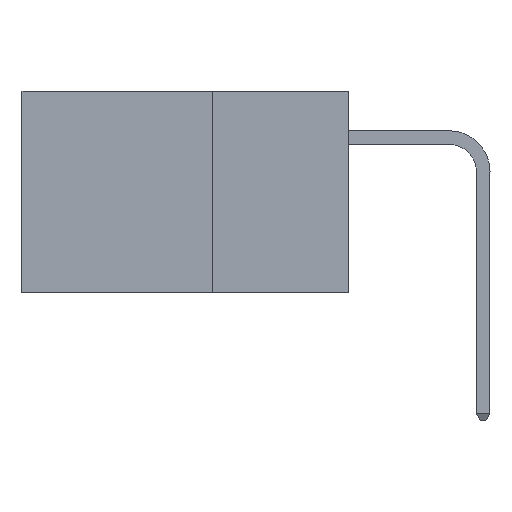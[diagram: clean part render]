
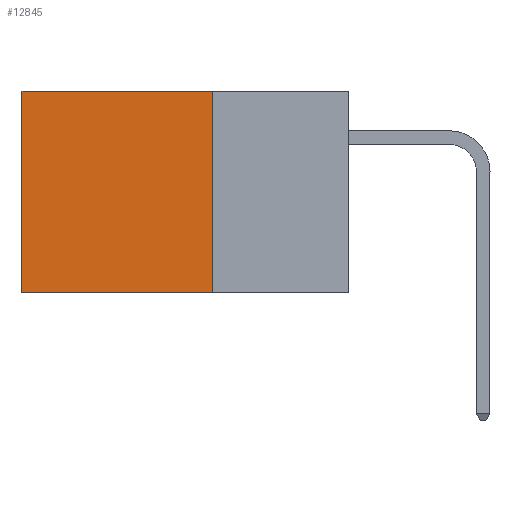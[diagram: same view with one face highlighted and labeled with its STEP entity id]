
A CAD part, left-side view. The second image highlights one B-rep face of the part: STEP entity #12845.
In plain terms, the highlighted planar face has unit normal (-1, 0, 0).
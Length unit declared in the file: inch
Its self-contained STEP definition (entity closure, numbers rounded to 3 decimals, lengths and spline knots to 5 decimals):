
#63 = LINE ( 'NONE', #13773, #2975 ) ;
#496 = DIRECTION ( 'NONE',  ( 0., 0., -1. ) ) ;
#1422 = VERTEX_POINT ( 'NONE', #14630 ) ;
#1431 = CARTESIAN_POINT ( 'NONE',  ( 0.2875, 0.25, 0. ) ) ;
#1717 = VERTEX_POINT ( 'NONE', #9365 ) ;
#2301 = PLANE ( 'NONE',  #8598 ) ;
#2401 = EDGE_CURVE ( 'NONE', #10542, #1717, #6745, .T. ) ;
#2464 = DIRECTION ( 'NONE',  ( 0., 1., 0. ) ) ;
#2975 = VECTOR ( 'NONE', #12651, 39.37008 ) ;
#3568 = DIRECTION ( 'NONE',  ( 0., 0., -1. ) ) ;
#4400 = LINE ( 'NONE', #12216, #13620 ) ;
#4548 = CARTESIAN_POINT ( 'NONE',  ( 0.2875, 0.6, 0. ) ) ;
#4964 = ORIENTED_EDGE ( 'NONE', *, *, #2401, .T. ) ;
#5554 = EDGE_CURVE ( 'NONE', #11391, #10542, #63, .T. ) ;
#5913 = CARTESIAN_POINT ( 'NONE',  ( 0.2875, 0.6, 0. ) ) ;
#6288 = ORIENTED_EDGE ( 'NONE', *, *, #10672, .F. ) ;
#6574 = VECTOR ( 'NONE', #10638, 39.37008 ) ;
#6745 = LINE ( 'NONE', #4548, #6574 ) ;
#6969 = ORIENTED_EDGE ( 'NONE', *, *, #9859, .F. ) ;
#7053 = ORIENTED_EDGE ( 'NONE', *, *, #5554, .T. ) ;
#7103 = VECTOR ( 'NONE', #496, 39.37008 ) ;
#7979 = CARTESIAN_POINT ( 'NONE',  ( 0.2875, 0.25, 0. ) ) ;
#8598 = AXIS2_PLACEMENT_3D ( 'NONE', #12011, #10877, #3568 ) ;
#9365 = CARTESIAN_POINT ( 'NONE',  ( 0.2875, 0.6, -0.37 ) ) ;
#9859 = EDGE_CURVE ( 'NONE', #11391, #1422, #13813, .T. ) ;
#10542 = VERTEX_POINT ( 'NONE', #5913 ) ;
#10638 = DIRECTION ( 'NONE',  ( 0., 0., -1. ) ) ;
#10672 = EDGE_CURVE ( 'NONE', #1422, #1717, #4400, .T. ) ;
#10877 = DIRECTION ( 'NONE',  ( 1., 0., 0. ) ) ;
#11391 = VERTEX_POINT ( 'NONE', #1431 ) ;
#12011 = CARTESIAN_POINT ( 'NONE',  ( 0.2875, 0.25, 0. ) ) ;
#12216 = CARTESIAN_POINT ( 'NONE',  ( 0.2875, 0.25, -0.37 ) ) ;
#12651 = DIRECTION ( 'NONE',  ( 0., 1., 0. ) ) ;
#12845 = ADVANCED_FACE ( 'NONE', ( #15487 ), #2301, .F. ) ;
#13620 = VECTOR ( 'NONE', #2464, 39.37008 ) ;
#13773 = CARTESIAN_POINT ( 'NONE',  ( 0.2875, 0.25, 0. ) ) ;
#13813 = LINE ( 'NONE', #7979, #7103 ) ;
#14007 = EDGE_LOOP ( 'NONE', ( #4964, #6288, #6969, #7053 ) ) ;
#14630 = CARTESIAN_POINT ( 'NONE',  ( 0.2875, 0.25, -0.37 ) ) ;
#15487 = FACE_OUTER_BOUND ( 'NONE', #14007, .T. ) ;
